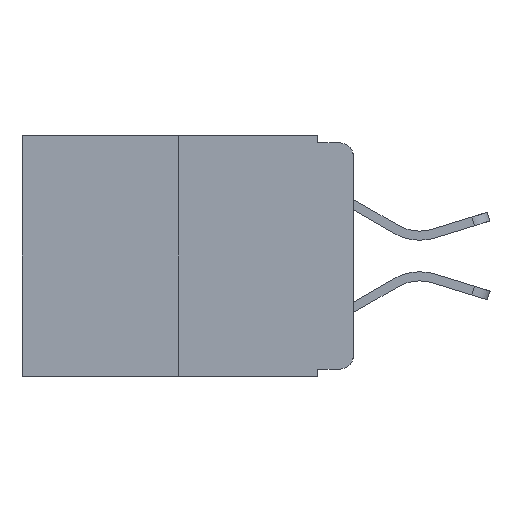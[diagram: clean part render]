
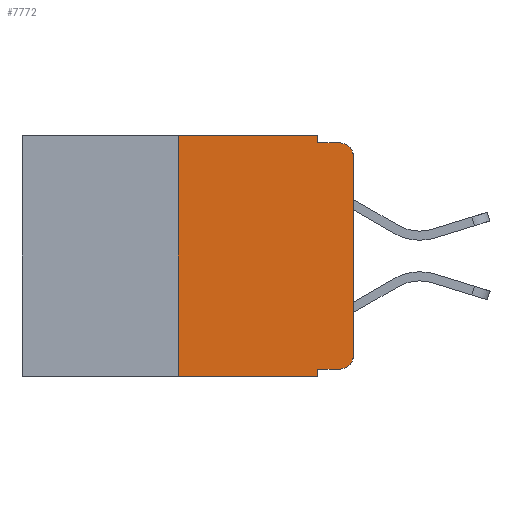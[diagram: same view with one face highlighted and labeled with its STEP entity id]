
A CAD part, left-side view. The second image highlights one B-rep face of the part: STEP entity #7772.
In plain terms, the highlighted planar face has unit normal (-1, 0, 0).
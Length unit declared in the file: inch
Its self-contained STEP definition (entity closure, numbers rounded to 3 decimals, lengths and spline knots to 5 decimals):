
#527 = ORIENTED_EDGE ( 'NONE', *, *, #6300, .T. ) ;
#581 = LINE ( 'NONE', #12157, #13611 ) ;
#1040 = DIRECTION ( 'NONE',  ( 0., 0., -1. ) ) ;
#1399 = VERTEX_POINT ( 'NONE', #9348 ) ;
#1470 = CARTESIAN_POINT ( 'NONE',  ( 0., 0., 0. ) ) ;
#2161 = EDGE_CURVE ( 'NONE', #9534, #9215, #3305, .T. ) ;
#2323 = DIRECTION ( 'NONE',  ( 0., -1., 0. ) ) ;
#2324 = ORIENTED_EDGE ( 'NONE', *, *, #22978, .T. ) ;
#2648 = ORIENTED_EDGE ( 'NONE', *, *, #4034, .F. ) ;
#3099 = ORIENTED_EDGE ( 'NONE', *, *, #7637, .F. ) ;
#3209 = EDGE_CURVE ( 'NONE', #21154, #14395, #22961, .T. ) ;
#3305 = LINE ( 'NONE', #13339, #23276 ) ;
#3437 = LINE ( 'NONE', #7770, #16396 ) ;
#3831 = CARTESIAN_POINT ( 'NONE',  ( 0., 0.02, -0.313 ) ) ;
#4012 = VECTOR ( 'NONE', #12954, 39.37008 ) ;
#4034 = EDGE_CURVE ( 'NONE', #13421, #12198, #10568, .T. ) ;
#4591 = FACE_OUTER_BOUND ( 'NONE', #4849, .T. ) ;
#4849 = EDGE_LOOP ( 'NONE', ( #16004, #15687, #14459, #20259, #3099, #12541, #527, #2648, #10961, #2324 ) ) ;
#4886 = CARTESIAN_POINT ( 'NONE',  ( 0., 0., -0.313 ) ) ;
#5432 = VECTOR ( 'NONE', #14957, 39.37008 ) ;
#6075 = DIRECTION ( 'NONE',  ( -1., 0., 0. ) ) ;
#6263 = CIRCLE ( 'NONE', #11561, 0.02 ) ;
#6300 = EDGE_CURVE ( 'NONE', #12543, #12198, #581, .T. ) ;
#6421 = DIRECTION ( 'NONE',  ( 0., -1., 0. ) ) ;
#6738 = CARTESIAN_POINT ( 'NONE',  ( 0., 0.02, -0.333 ) ) ;
#7637 = EDGE_CURVE ( 'NONE', #12900, #9534, #9587, .T. ) ;
#7672 = DIRECTION ( 'NONE',  ( 0., 0., -1. ) ) ;
#7770 = CARTESIAN_POINT ( 'NONE',  ( 0., 0.051, -0.333 ) ) ;
#7772 = ADVANCED_FACE ( 'NONE', ( #4591 ), #19853, .F. ) ;
#8259 = EDGE_CURVE ( 'NONE', #9215, #1399, #21873, .T. ) ;
#8272 = DIRECTION ( 'NONE',  ( 0., 0., -1. ) ) ;
#9046 = CIRCLE ( 'NONE', #22018, 0.02 ) ;
#9215 = VERTEX_POINT ( 'NONE', #13242 ) ;
#9348 = CARTESIAN_POINT ( 'NONE',  ( 0., 0.02, -0.01 ) ) ;
#9534 = VERTEX_POINT ( 'NONE', #11187 ) ;
#9587 = LINE ( 'NONE', #19733, #17389 ) ;
#10168 = CARTESIAN_POINT ( 'NONE',  ( 0., 0.25, -0.343 ) ) ;
#10469 = CARTESIAN_POINT ( 'NONE',  ( 0., 0.051, -0.343 ) ) ;
#10568 = LINE ( 'NONE', #18312, #13176 ) ;
#10725 = VECTOR ( 'NONE', #17941, 39.37008 ) ;
#10777 = VERTEX_POINT ( 'NONE', #6738 ) ;
#10961 = ORIENTED_EDGE ( 'NONE', *, *, #25111, .T. ) ;
#11187 = CARTESIAN_POINT ( 'NONE',  ( 0., 0.051, 0. ) ) ;
#11561 = AXIS2_PLACEMENT_3D ( 'NONE', #19435, #6075, #8272 ) ;
#11781 = CARTESIAN_POINT ( 'NONE',  ( 0., 0.25, 0. ) ) ;
#12157 = CARTESIAN_POINT ( 'NONE',  ( 0., 0.473, -0.343 ) ) ;
#12198 = VERTEX_POINT ( 'NONE', #10469 ) ;
#12541 = ORIENTED_EDGE ( 'NONE', *, *, #24756, .F. ) ;
#12543 = VERTEX_POINT ( 'NONE', #10168 ) ;
#12833 = CARTESIAN_POINT ( 'NONE',  ( 0., 0.051, -0.01 ) ) ;
#12900 = VERTEX_POINT ( 'NONE', #11781 ) ;
#12954 = DIRECTION ( 'NONE',  ( 0., -1., 0. ) ) ;
#13176 = VECTOR ( 'NONE', #17938, 39.37008 ) ;
#13242 = CARTESIAN_POINT ( 'NONE',  ( 0., 0.051, -0.01 ) ) ;
#13339 = CARTESIAN_POINT ( 'NONE',  ( 0., 0.051, 0. ) ) ;
#13421 = VERTEX_POINT ( 'NONE', #25059 ) ;
#13611 = VECTOR ( 'NONE', #6421, 39.37008 ) ;
#13752 = DIRECTION ( 'NONE',  ( -1., 0., 0. ) ) ;
#13863 = CARTESIAN_POINT ( 'NONE',  ( 0., 0., -0.03 ) ) ;
#14025 = CARTESIAN_POINT ( 'NONE',  ( 0., 0.25, 0. ) ) ;
#14352 = EDGE_CURVE ( 'NONE', #14395, #1399, #6263, .T. ) ;
#14395 = VERTEX_POINT ( 'NONE', #13863 ) ;
#14459 = ORIENTED_EDGE ( 'NONE', *, *, #8259, .F. ) ;
#14957 = DIRECTION ( 'NONE',  ( 0., 0., 1. ) ) ;
#15004 = DIRECTION ( 'NONE',  ( 0., 0., -1. ) ) ;
#15687 = ORIENTED_EDGE ( 'NONE', *, *, #14352, .T. ) ;
#16004 = ORIENTED_EDGE ( 'NONE', *, *, #3209, .T. ) ;
#16396 = VECTOR ( 'NONE', #19316, 39.37008 ) ;
#17389 = VECTOR ( 'NONE', #2323, 39.37008 ) ;
#17809 = LINE ( 'NONE', #14025, #10725 ) ;
#17938 = DIRECTION ( 'NONE',  ( 0., 0., -1. ) ) ;
#17941 = DIRECTION ( 'NONE',  ( 0., 0., 1. ) ) ;
#18312 = CARTESIAN_POINT ( 'NONE',  ( 0., 0.051, 0. ) ) ;
#18461 = CARTESIAN_POINT ( 'NONE',  ( 0., 0.473, 0. ) ) ;
#19027 = AXIS2_PLACEMENT_3D ( 'NONE', #18461, #22290, #1040 ) ;
#19316 = DIRECTION ( 'NONE',  ( 0., -1., 0. ) ) ;
#19435 = CARTESIAN_POINT ( 'NONE',  ( 0., 0.02, -0.03 ) ) ;
#19733 = CARTESIAN_POINT ( 'NONE',  ( 0., 0.473, 0. ) ) ;
#19853 = PLANE ( 'NONE',  #19027 ) ;
#20259 = ORIENTED_EDGE ( 'NONE', *, *, #2161, .F. ) ;
#21154 = VERTEX_POINT ( 'NONE', #4886 ) ;
#21873 = LINE ( 'NONE', #12833, #4012 ) ;
#22018 = AXIS2_PLACEMENT_3D ( 'NONE', #3831, #13752, #7672 ) ;
#22290 = DIRECTION ( 'NONE',  ( 1., 0., 0. ) ) ;
#22961 = LINE ( 'NONE', #1470, #5432 ) ;
#22978 = EDGE_CURVE ( 'NONE', #10777, #21154, #9046, .T. ) ;
#23276 = VECTOR ( 'NONE', #15004, 39.37008 ) ;
#24756 = EDGE_CURVE ( 'NONE', #12543, #12900, #17809, .T. ) ;
#25059 = CARTESIAN_POINT ( 'NONE',  ( 0., 0.051, -0.333 ) ) ;
#25111 = EDGE_CURVE ( 'NONE', #13421, #10777, #3437, .T. ) ;
